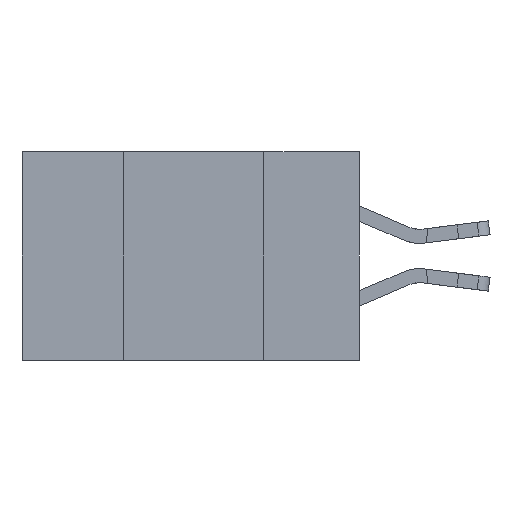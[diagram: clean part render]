
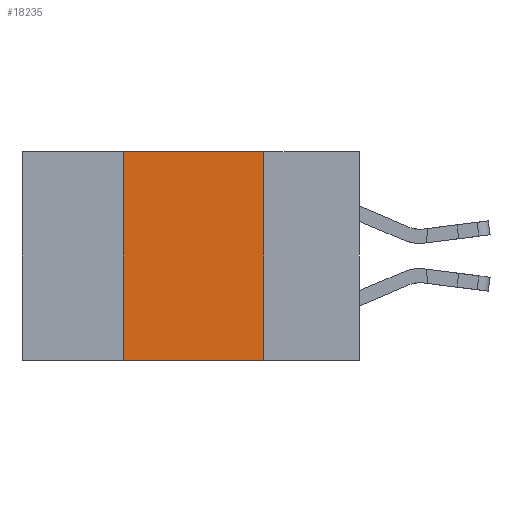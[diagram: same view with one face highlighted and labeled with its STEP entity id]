
A CAD part, left-side view. The second image highlights one B-rep face of the part: STEP entity #18235.
In plain terms, the highlighted planar face has unit normal (-1, 0, 0).
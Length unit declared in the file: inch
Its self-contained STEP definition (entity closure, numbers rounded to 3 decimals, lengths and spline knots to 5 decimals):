
#187 = VECTOR ( 'NONE', #19995, 39.37008 ) ;
#353 = PLANE ( 'NONE',  #10377 ) ;
#2967 = DIRECTION ( 'NONE',  ( 0., 0., 1. ) ) ;
#3000 = DIRECTION ( 'NONE',  ( 0., 0., -1. ) ) ;
#3264 = ORIENTED_EDGE ( 'NONE', *, *, #6071, .T. ) ;
#3497 = CARTESIAN_POINT ( 'NONE',  ( 0., 0.17, -0.37 ) ) ;
#3753 = ORIENTED_EDGE ( 'NONE', *, *, #20753, .F. ) ;
#4277 = DIRECTION ( 'NONE',  ( 0., 0., -1. ) ) ;
#4660 = VERTEX_POINT ( 'NONE', #7269 ) ;
#5095 = CARTESIAN_POINT ( 'NONE',  ( 0., 0.6, -0.37 ) ) ;
#5482 = CARTESIAN_POINT ( 'NONE',  ( 0., 0.6, 0. ) ) ;
#5936 = CARTESIAN_POINT ( 'NONE',  ( 0., 0.17, 0. ) ) ;
#6071 = EDGE_CURVE ( 'NONE', #6492, #23703, #20239, .T. ) ;
#6492 = VERTEX_POINT ( 'NONE', #24062 ) ;
#6765 = CARTESIAN_POINT ( 'NONE',  ( 0., 0.42, 0. ) ) ;
#7269 = CARTESIAN_POINT ( 'NONE',  ( 0., 0.42, 0. ) ) ;
#8906 = ORIENTED_EDGE ( 'NONE', *, *, #22265, .F. ) ;
#10377 = AXIS2_PLACEMENT_3D ( 'NONE', #13617, #15505, #4277 ) ;
#10475 = EDGE_LOOP ( 'NONE', ( #11086, #3753, #8906, #3264 ) ) ;
#11086 = ORIENTED_EDGE ( 'NONE', *, *, #23532, .F. ) ;
#12401 = VECTOR ( 'NONE', #2967, 39.37008 ) ;
#13071 = DIRECTION ( 'NONE',  ( 0., -1., 0. ) ) ;
#13617 = CARTESIAN_POINT ( 'NONE',  ( 0., 0.6, 0. ) ) ;
#15505 = DIRECTION ( 'NONE',  ( 1., 0., 0. ) ) ;
#16973 = LINE ( 'NONE', #18016, #20724 ) ;
#17154 = VECTOR ( 'NONE', #13071, 39.37008 ) ;
#17730 = LINE ( 'NONE', #5482, #17154 ) ;
#18016 = CARTESIAN_POINT ( 'NONE',  ( 0., 0.17, 0. ) ) ;
#18235 = ADVANCED_FACE ( 'NONE', ( #18385 ), #353, .F. ) ;
#18385 = FACE_OUTER_BOUND ( 'NONE', #10475, .T. ) ;
#19995 = DIRECTION ( 'NONE',  ( 0., -1., 0. ) ) ;
#20239 = LINE ( 'NONE', #5095, #187 ) ;
#20724 = VECTOR ( 'NONE', #3000, 39.37008 ) ;
#20753 = EDGE_CURVE ( 'NONE', #4660, #21965, #17730, .T. ) ;
#21965 = VERTEX_POINT ( 'NONE', #5936 ) ;
#22265 = EDGE_CURVE ( 'NONE', #6492, #4660, #22864, .T. ) ;
#22864 = LINE ( 'NONE', #6765, #12401 ) ;
#23532 = EDGE_CURVE ( 'NONE', #21965, #23703, #16973, .T. ) ;
#23703 = VERTEX_POINT ( 'NONE', #3497 ) ;
#24062 = CARTESIAN_POINT ( 'NONE',  ( 0., 0.42, -0.37 ) ) ;
